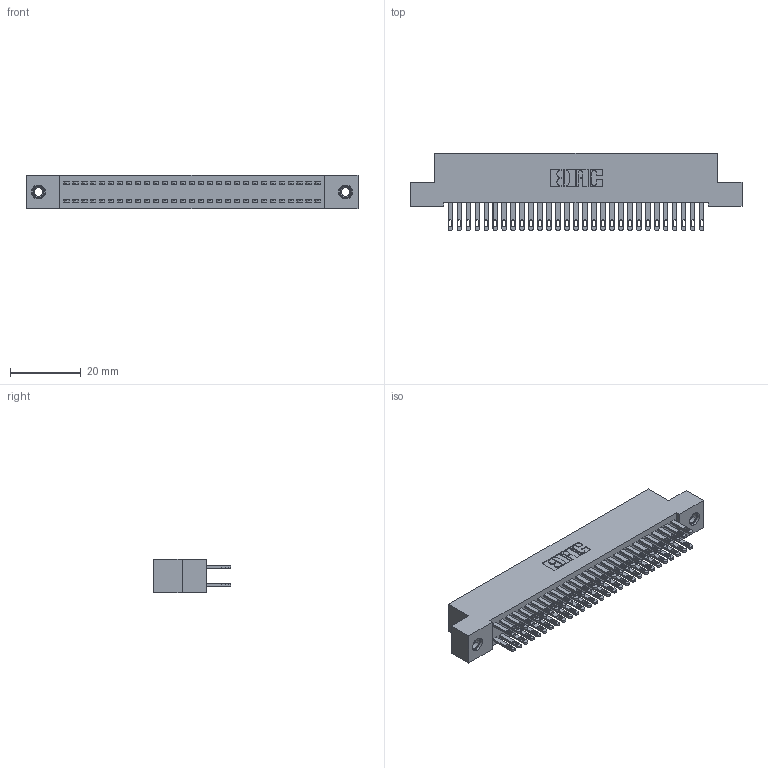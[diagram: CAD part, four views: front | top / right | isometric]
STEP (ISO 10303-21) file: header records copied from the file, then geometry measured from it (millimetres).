
FILE_DESCRIPTION (( 'STEP AP203' ), '1' );
FILE_NAME ('342-058-500-207.STEP', '2018-08-13T04:50:33', ( '' ), ( '' ), 'SwSTEP 2.0', 'SolidWorks 2016', '' );
FILE_SCHEMA (( 'CONFIG_CONTROL_DESIGN' ));
Length unit declared in the file: inch
Products named in the file (4): 342 Part_TI; 345-292-001_345-293-100; 345-250-001_345-250-005-103; 342-058-500-207
Assembly tree (61 placements, depth 2):
  342-058-500-207
    342 Part_TI
    345-292-001_345-293-100  x58
    345-250-001_345-250-005-103  x2
Bounding box: 93.98 x 21.85 x 9.4 mm (x, y, z)
Volume: 8547.1 mm3; surface area: 14173.3 mm2
Topology: 61 solids, 61 shells, 2954 faces, 8961 edges, 5966 vertices
Faces by surface type: plane 1838, cylinder 1100, cone 12, torus 4
Entity records: 21322 total; most frequent: CARTESIAN_POINT 3529, ORIENTED_EDGE 3458, DIRECTION 3071, EDGE_CURVE 1729, VECTOR 1577, LINE 1577, VERTEX_POINT 1148, AXIS2_PLACEMENT_3D 747
